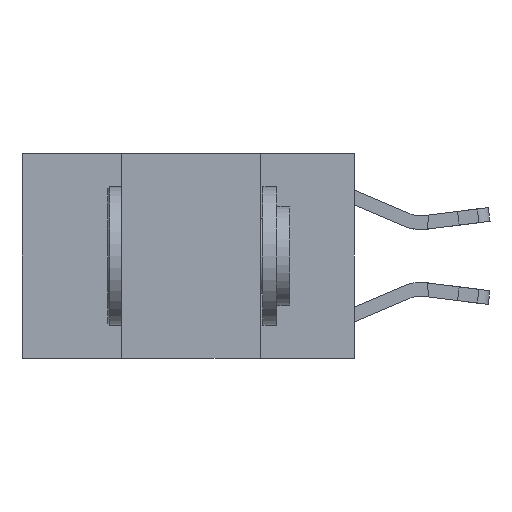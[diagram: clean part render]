
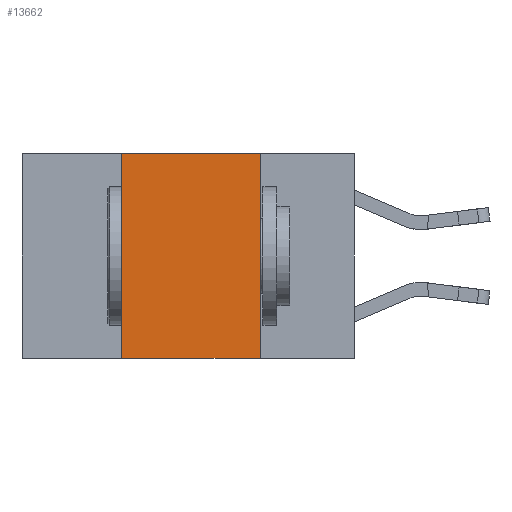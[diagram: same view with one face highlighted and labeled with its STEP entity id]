
A CAD part, left-side view. The second image highlights one B-rep face of the part: STEP entity #13662.
In plain terms, the highlighted planar face has unit normal (-1, 0, 0).
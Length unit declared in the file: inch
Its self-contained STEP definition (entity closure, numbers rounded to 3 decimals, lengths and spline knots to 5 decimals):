
#105 = EDGE_LOOP ( 'NONE', ( #18741, #6182, #19757, #2759 ) ) ;
#195 = LINE ( 'NONE', #1434, #4158 ) ;
#364 = AXIS2_PLACEMENT_3D ( 'NONE', #13602, #18457, #8667 ) ;
#690 = EDGE_CURVE ( 'NONE', #3646, #3552, #3216, .T. ) ;
#1434 = CARTESIAN_POINT ( 'NONE',  ( 0., 0.6, 0. ) ) ;
#1797 = CARTESIAN_POINT ( 'NONE',  ( 0., 0.42, 0. ) ) ;
#2759 = ORIENTED_EDGE ( 'NONE', *, *, #3386, .T. ) ;
#3216 = LINE ( 'NONE', #19740, #19693 ) ;
#3386 = EDGE_CURVE ( 'NONE', #13271, #3552, #4964, .T. ) ;
#3552 = VERTEX_POINT ( 'NONE', #14098 ) ;
#3646 = VERTEX_POINT ( 'NONE', #19083 ) ;
#3728 = LINE ( 'NONE', #14188, #16432 ) ;
#4158 = VECTOR ( 'NONE', #21073, 39.37008 ) ;
#4964 = LINE ( 'NONE', #20860, #13311 ) ;
#6060 = CARTESIAN_POINT ( 'NONE',  ( 0., 0.42, -0.37 ) ) ;
#6182 = ORIENTED_EDGE ( 'NONE', *, *, #12088, .F. ) ;
#6994 = PLANE ( 'NONE',  #364 ) ;
#8667 = DIRECTION ( 'NONE',  ( 0., 0., -1. ) ) ;
#11877 = DIRECTION ( 'NONE',  ( 0., -1., 0. ) ) ;
#12088 = EDGE_CURVE ( 'NONE', #13596, #3646, #195, .T. ) ;
#13271 = VERTEX_POINT ( 'NONE', #6060 ) ;
#13311 = VECTOR ( 'NONE', #11877, 39.37008 ) ;
#13596 = VERTEX_POINT ( 'NONE', #1797 ) ;
#13602 = CARTESIAN_POINT ( 'NONE',  ( 0., 0.6, 0. ) ) ;
#13662 = ADVANCED_FACE ( 'NONE', ( #18051 ), #6994, .F. ) ;
#14098 = CARTESIAN_POINT ( 'NONE',  ( 0., 0.17, -0.37 ) ) ;
#14188 = CARTESIAN_POINT ( 'NONE',  ( 0., 0.42, 0. ) ) ;
#15800 = DIRECTION ( 'NONE',  ( 0., 0., 1. ) ) ;
#16432 = VECTOR ( 'NONE', #15800, 39.37008 ) ;
#16696 = EDGE_CURVE ( 'NONE', #13271, #13596, #3728, .T. ) ;
#18051 = FACE_OUTER_BOUND ( 'NONE', #105, .T. ) ;
#18457 = DIRECTION ( 'NONE',  ( 1., 0., 0. ) ) ;
#18741 = ORIENTED_EDGE ( 'NONE', *, *, #690, .F. ) ;
#19083 = CARTESIAN_POINT ( 'NONE',  ( 0., 0.17, 0. ) ) ;
#19691 = DIRECTION ( 'NONE',  ( 0., 0., -1. ) ) ;
#19693 = VECTOR ( 'NONE', #19691, 39.37008 ) ;
#19740 = CARTESIAN_POINT ( 'NONE',  ( 0., 0.17, 0. ) ) ;
#19757 = ORIENTED_EDGE ( 'NONE', *, *, #16696, .F. ) ;
#20860 = CARTESIAN_POINT ( 'NONE',  ( 0., 0.6, -0.37 ) ) ;
#21073 = DIRECTION ( 'NONE',  ( 0., -1., 0. ) ) ;
